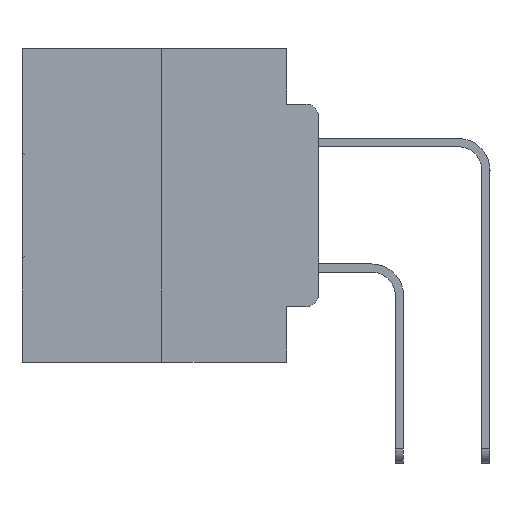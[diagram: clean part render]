
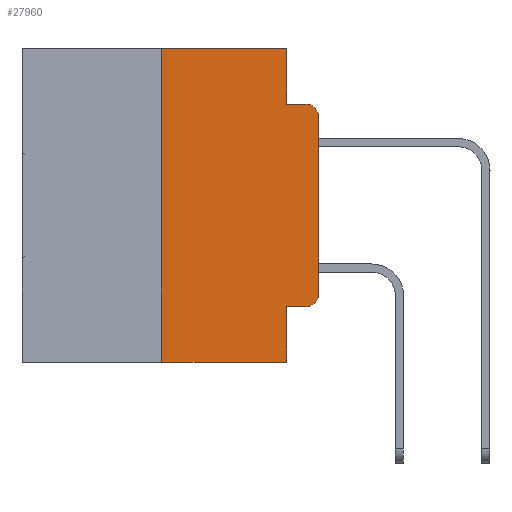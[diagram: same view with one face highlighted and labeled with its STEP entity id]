
A CAD part, left-side view. The second image highlights one B-rep face of the part: STEP entity #27960.
In plain terms, the highlighted planar face has unit normal (-1, 0, 0).
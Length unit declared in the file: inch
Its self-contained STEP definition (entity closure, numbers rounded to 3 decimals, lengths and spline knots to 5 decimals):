
#350 = VECTOR ( 'NONE', #31824, 39.37008 ) ;
#824 = ORIENTED_EDGE ( 'NONE', *, *, #28700, .F. ) ;
#1055 = LINE ( 'NONE', #19210, #21726 ) ;
#1806 = VERTEX_POINT ( 'NONE', #28564 ) ;
#1870 = ORIENTED_EDGE ( 'NONE', *, *, #3282, .T. ) ;
#1979 = EDGE_CURVE ( 'NONE', #12458, #25766, #1055, .T. ) ;
#2195 = CARTESIAN_POINT ( 'NONE',  ( 0., 0.051, 0. ) ) ;
#3182 = CARTESIAN_POINT ( 'NONE',  ( 0., 0.02, -0.4115 ) ) ;
#3282 = EDGE_CURVE ( 'NONE', #18267, #12057, #5895, .T. ) ;
#3326 = VECTOR ( 'NONE', #6000, 39.37008 ) ;
#3950 = CARTESIAN_POINT ( 'NONE',  ( 0., 0.02, -0.3915 ) ) ;
#4199 = CARTESIAN_POINT ( 'NONE',  ( 0., 0.25, 0. ) ) ;
#4321 = EDGE_CURVE ( 'NONE', #12057, #10603, #9383, .T. ) ;
#4674 = LINE ( 'NONE', #30826, #7810 ) ;
#4759 = VECTOR ( 'NONE', #7182, 39.37008 ) ;
#4791 = VERTEX_POINT ( 'NONE', #16898 ) ;
#5745 = PLANE ( 'NONE',  #7371 ) ;
#5895 = LINE ( 'NONE', #22142, #4759 ) ;
#5957 = ORIENTED_EDGE ( 'NONE', *, *, #4321, .T. ) ;
#6000 = DIRECTION ( 'NONE',  ( 0., 0., -1. ) ) ;
#6081 = CARTESIAN_POINT ( 'NONE',  ( 0., 0.473, 0. ) ) ;
#7182 = DIRECTION ( 'NONE',  ( 0., -1., 0. ) ) ;
#7238 = LINE ( 'NONE', #25990, #3326 ) ;
#7371 = AXIS2_PLACEMENT_3D ( 'NONE', #6081, #25637, #13432 ) ;
#7747 = ORIENTED_EDGE ( 'NONE', *, *, #9842, .F. ) ;
#7810 = VECTOR ( 'NONE', #25805, 39.37008 ) ;
#8737 = CARTESIAN_POINT ( 'NONE',  ( 0., 0.473, 0. ) ) ;
#9023 = CARTESIAN_POINT ( 'NONE',  ( 0., 0.051, -0.4115 ) ) ;
#9284 = CARTESIAN_POINT ( 'NONE',  ( 0., 0.25, -0.5 ) ) ;
#9383 = CIRCLE ( 'NONE', #12524, 0.02 ) ;
#9429 = EDGE_CURVE ( 'NONE', #10603, #1806, #29774, .T. ) ;
#9698 = ORIENTED_EDGE ( 'NONE', *, *, #1979, .T. ) ;
#9842 = EDGE_CURVE ( 'NONE', #18267, #25766, #10671, .T. ) ;
#10578 = CARTESIAN_POINT ( 'NONE',  ( 0., 0.051, -0.0885 ) ) ;
#10603 = VERTEX_POINT ( 'NONE', #24951 ) ;
#10671 = LINE ( 'NONE', #2195, #25070 ) ;
#12057 = VERTEX_POINT ( 'NONE', #3182 ) ;
#12368 = EDGE_LOOP ( 'NONE', ( #15094, #18224, #824, #16694, #19229, #15731, #9698, #7747, #1870, #5957 ) ) ;
#12458 = VERTEX_POINT ( 'NONE', #9284 ) ;
#12524 = AXIS2_PLACEMENT_3D ( 'NONE', #3950, #21426, #14226 ) ;
#12840 = VERTEX_POINT ( 'NONE', #15504 ) ;
#13118 = CARTESIAN_POINT ( 'NONE',  ( 0., 0., 0. ) ) ;
#13432 = DIRECTION ( 'NONE',  ( 0., 0., -1. ) ) ;
#14226 = DIRECTION ( 'NONE',  ( 0., 0., -1. ) ) ;
#15059 = EDGE_CURVE ( 'NONE', #1806, #12840, #22391, .T. ) ;
#15094 = ORIENTED_EDGE ( 'NONE', *, *, #9429, .T. ) ;
#15504 = CARTESIAN_POINT ( 'NONE',  ( 0., 0.02, -0.0885 ) ) ;
#15731 = ORIENTED_EDGE ( 'NONE', *, *, #26938, .F. ) ;
#16196 = CARTESIAN_POINT ( 'NONE',  ( 0., 0.051, -0.5 ) ) ;
#16694 = ORIENTED_EDGE ( 'NONE', *, *, #19270, .F. ) ;
#16721 = CARTESIAN_POINT ( 'NONE',  ( 0., 0.051, 0. ) ) ;
#16898 = CARTESIAN_POINT ( 'NONE',  ( 0., 0.25, 0. ) ) ;
#17042 = VERTEX_POINT ( 'NONE', #16721 ) ;
#18224 = ORIENTED_EDGE ( 'NONE', *, *, #15059, .T. ) ;
#18267 = VERTEX_POINT ( 'NONE', #9023 ) ;
#18551 = LINE ( 'NONE', #8737, #25190 ) ;
#19040 = DIRECTION ( 'NONE',  ( -1., 0., 0. ) ) ;
#19210 = CARTESIAN_POINT ( 'NONE',  ( 0., 0.473, -0.5 ) ) ;
#19229 = ORIENTED_EDGE ( 'NONE', *, *, #23272, .F. ) ;
#19270 = EDGE_CURVE ( 'NONE', #17042, #19899, #7238, .T. ) ;
#19899 = VERTEX_POINT ( 'NONE', #10578 ) ;
#19967 = DIRECTION ( 'NONE',  ( 0., -1., 0. ) ) ;
#20955 = DIRECTION ( 'NONE',  ( 0., 0., 1. ) ) ;
#21426 = DIRECTION ( 'NONE',  ( -1., 0., 0. ) ) ;
#21726 = VECTOR ( 'NONE', #19967, 39.37008 ) ;
#22142 = CARTESIAN_POINT ( 'NONE',  ( 0., 0.051, -0.4115 ) ) ;
#22391 = CIRCLE ( 'NONE', #24219, 0.02 ) ;
#23272 = EDGE_CURVE ( 'NONE', #4791, #17042, #18551, .T. ) ;
#23708 = DIRECTION ( 'NONE',  ( 0., -1., 0. ) ) ;
#24219 = AXIS2_PLACEMENT_3D ( 'NONE', #26338, #19040, #28842 ) ;
#24951 = CARTESIAN_POINT ( 'NONE',  ( 0., 0., -0.3915 ) ) ;
#25070 = VECTOR ( 'NONE', #27480, 39.37008 ) ;
#25190 = VECTOR ( 'NONE', #23708, 39.37008 ) ;
#25637 = DIRECTION ( 'NONE',  ( 1., 0., 0. ) ) ;
#25766 = VERTEX_POINT ( 'NONE', #16196 ) ;
#25805 = DIRECTION ( 'NONE',  ( 0., -1., 0. ) ) ;
#25990 = CARTESIAN_POINT ( 'NONE',  ( 0., 0.051, 0. ) ) ;
#26338 = CARTESIAN_POINT ( 'NONE',  ( 0., 0.02, -0.1085 ) ) ;
#26639 = VECTOR ( 'NONE', #20955, 39.37008 ) ;
#26938 = EDGE_CURVE ( 'NONE', #12458, #4791, #29255, .T. ) ;
#27480 = DIRECTION ( 'NONE',  ( 0., 0., -1. ) ) ;
#27960 = ADVANCED_FACE ( 'NONE', ( #28383 ), #5745, .F. ) ;
#28383 = FACE_OUTER_BOUND ( 'NONE', #12368, .T. ) ;
#28564 = CARTESIAN_POINT ( 'NONE',  ( 0., 0., -0.1085 ) ) ;
#28700 = EDGE_CURVE ( 'NONE', #19899, #12840, #4674, .T. ) ;
#28842 = DIRECTION ( 'NONE',  ( 0., 0., -1. ) ) ;
#29255 = LINE ( 'NONE', #4199, #350 ) ;
#29774 = LINE ( 'NONE', #13118, #26639 ) ;
#30826 = CARTESIAN_POINT ( 'NONE',  ( 0., 0.051, -0.0885 ) ) ;
#31824 = DIRECTION ( 'NONE',  ( 0., 0., 1. ) ) ;
